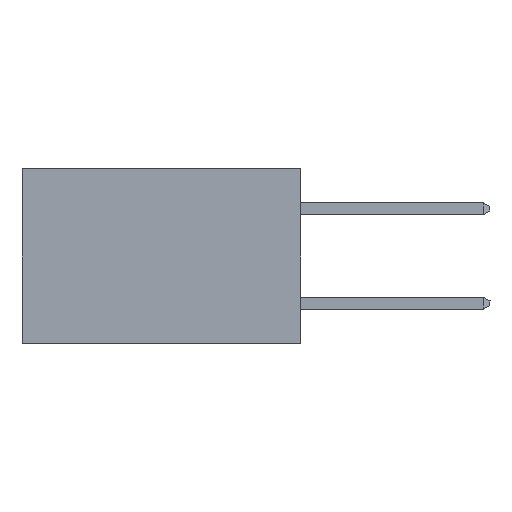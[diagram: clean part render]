
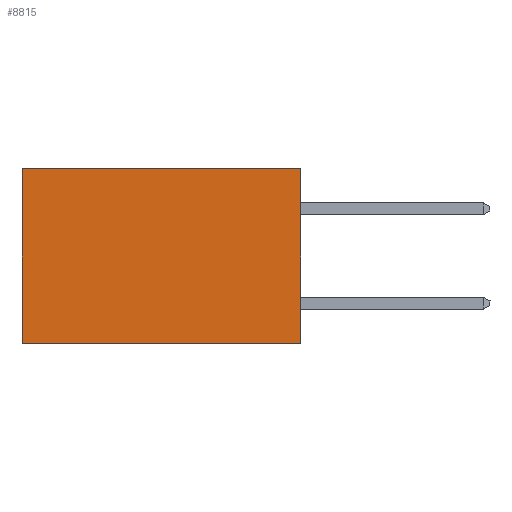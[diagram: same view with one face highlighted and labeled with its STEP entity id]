
A CAD part, left-side view. The second image highlights one B-rep face of the part: STEP entity #8815.
In plain terms, the highlighted planar face has unit normal (-1, 0, 0).
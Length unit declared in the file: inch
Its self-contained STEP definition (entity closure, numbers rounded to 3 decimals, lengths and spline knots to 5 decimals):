
#428 = VECTOR ( 'NONE', #12915, 39.37008 ) ;
#1126 = CARTESIAN_POINT ( 'NONE',  ( 0.277, 0., 0. ) ) ;
#1421 = ORIENTED_EDGE ( 'NONE', *, *, #2358, .T. ) ;
#1721 = ORIENTED_EDGE ( 'NONE', *, *, #20516, .F. ) ;
#2248 = DIRECTION ( 'NONE',  ( 1., 0., 0. ) ) ;
#2358 = EDGE_CURVE ( 'NONE', #21318, #10292, #33761, .T. ) ;
#3172 = VERTEX_POINT ( 'NONE', #21620 ) ;
#4008 = DIRECTION ( 'NONE',  ( 0., 0., -1. ) ) ;
#5618 = VERTEX_POINT ( 'NONE', #1126 ) ;
#6286 = CARTESIAN_POINT ( 'NONE',  ( 0.277, 0.59, 0. ) ) ;
#6903 = CARTESIAN_POINT ( 'NONE',  ( 0.277, 0.59, -0.37 ) ) ;
#6938 = VECTOR ( 'NONE', #4008, 39.37008 ) ;
#7947 = DIRECTION ( 'NONE',  ( 0., 1., 0. ) ) ;
#8122 = ORIENTED_EDGE ( 'NONE', *, *, #29482, .F. ) ;
#8815 = ADVANCED_FACE ( 'NONE', ( #23357 ), #34462, .F. ) ;
#10292 = VERTEX_POINT ( 'NONE', #24338 ) ;
#10904 = LINE ( 'NONE', #22136, #24427 ) ;
#12915 = DIRECTION ( 'NONE',  ( 0., 0., -1. ) ) ;
#14062 = LINE ( 'NONE', #29033, #428 ) ;
#15143 = EDGE_LOOP ( 'NONE', ( #1421, #1721, #8122, #34480 ) ) ;
#18549 = CARTESIAN_POINT ( 'NONE',  ( 0.277, 0., -0.37 ) ) ;
#20418 = VECTOR ( 'NONE', #7947, 39.37008 ) ;
#20516 = EDGE_CURVE ( 'NONE', #3172, #10292, #10904, .T. ) ;
#21256 = LINE ( 'NONE', #29480, #20418 ) ;
#21292 = DIRECTION ( 'NONE',  ( 0., 0., -1. ) ) ;
#21318 = VERTEX_POINT ( 'NONE', #6286 ) ;
#21620 = CARTESIAN_POINT ( 'NONE',  ( 0.277, 0., -0.37 ) ) ;
#22136 = CARTESIAN_POINT ( 'NONE',  ( 0.277, 0., -0.37 ) ) ;
#23349 = AXIS2_PLACEMENT_3D ( 'NONE', #18549, #2248, #21292 ) ;
#23357 = FACE_OUTER_BOUND ( 'NONE', #15143, .T. ) ;
#23715 = EDGE_CURVE ( 'NONE', #5618, #21318, #21256, .T. ) ;
#24338 = CARTESIAN_POINT ( 'NONE',  ( 0.277, 0.59, -0.37 ) ) ;
#24427 = VECTOR ( 'NONE', #24812, 39.37008 ) ;
#24812 = DIRECTION ( 'NONE',  ( 0., 1., 0. ) ) ;
#29033 = CARTESIAN_POINT ( 'NONE',  ( 0.277, 0., -0.37 ) ) ;
#29480 = CARTESIAN_POINT ( 'NONE',  ( 0.277, 0., 0. ) ) ;
#29482 = EDGE_CURVE ( 'NONE', #5618, #3172, #14062, .T. ) ;
#33761 = LINE ( 'NONE', #6903, #6938 ) ;
#34462 = PLANE ( 'NONE',  #23349 ) ;
#34480 = ORIENTED_EDGE ( 'NONE', *, *, #23715, .T. ) ;
